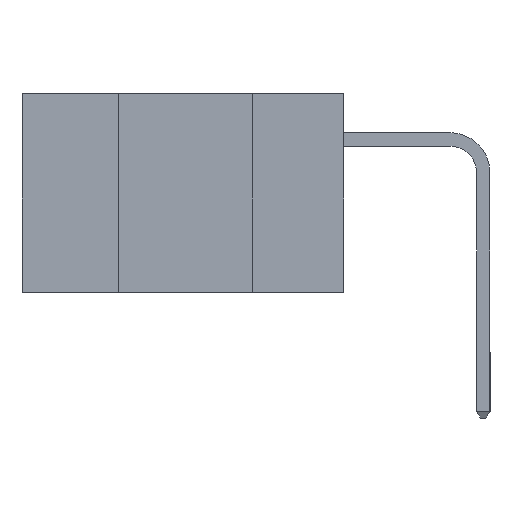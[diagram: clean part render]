
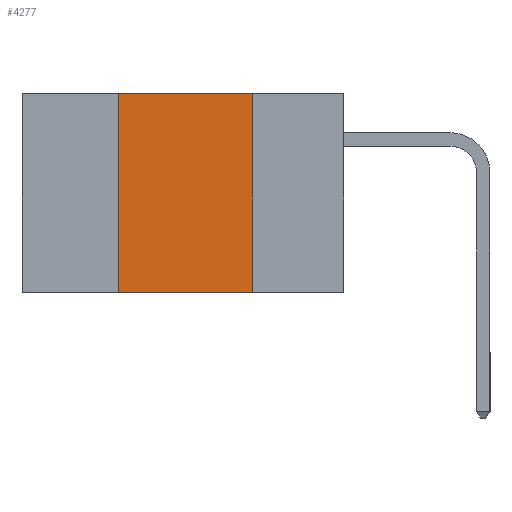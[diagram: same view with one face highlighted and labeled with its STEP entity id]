
A CAD part, left-side view. The second image highlights one B-rep face of the part: STEP entity #4277.
In plain terms, the highlighted planar face has unit normal (-1, 0, 0).
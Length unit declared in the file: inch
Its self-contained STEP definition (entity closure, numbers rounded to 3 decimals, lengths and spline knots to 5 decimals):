
#91 = LINE ( 'NONE', #2600, #12631 ) ;
#205 = EDGE_CURVE ( 'NONE', #9719, #13048, #2115, .T. ) ;
#1050 = DIRECTION ( 'NONE',  ( 0., 0., -1. ) ) ;
#1106 = CARTESIAN_POINT ( 'NONE',  ( 0., 0.17, 0. ) ) ;
#2115 = LINE ( 'NONE', #5083, #13080 ) ;
#2322 = CARTESIAN_POINT ( 'NONE',  ( 0., 0.42, 0. ) ) ;
#2352 = CARTESIAN_POINT ( 'NONE',  ( 0., 0.6, 0. ) ) ;
#2404 = DIRECTION ( 'NONE',  ( 1., 0., 0. ) ) ;
#2505 = ORIENTED_EDGE ( 'NONE', *, *, #5568, .F. ) ;
#2600 = CARTESIAN_POINT ( 'NONE',  ( 0., 0.6, 0. ) ) ;
#3003 = EDGE_CURVE ( 'NONE', #3076, #13048, #10635, .T. ) ;
#3076 = VERTEX_POINT ( 'NONE', #4480 ) ;
#3964 = CARTESIAN_POINT ( 'NONE',  ( 0., 0.42, -0.37 ) ) ;
#4085 = FACE_OUTER_BOUND ( 'NONE', #6163, .T. ) ;
#4277 = ADVANCED_FACE ( 'NONE', ( #4085 ), #10495, .F. ) ;
#4480 = CARTESIAN_POINT ( 'NONE',  ( 0., 0.17, 0. ) ) ;
#4756 = DIRECTION ( 'NONE',  ( 0., -1., 0. ) ) ;
#5083 = CARTESIAN_POINT ( 'NONE',  ( 0., 0.6, -0.37 ) ) ;
#5568 = EDGE_CURVE ( 'NONE', #8597, #3076, #91, .T. ) ;
#5594 = ORIENTED_EDGE ( 'NONE', *, *, #3003, .F. ) ;
#5931 = VECTOR ( 'NONE', #10267, 39.37008 ) ;
#6163 = EDGE_LOOP ( 'NONE', ( #5594, #2505, #7338, #10912 ) ) ;
#7194 = LINE ( 'NONE', #2322, #5931 ) ;
#7338 = ORIENTED_EDGE ( 'NONE', *, *, #8689, .F. ) ;
#7370 = DIRECTION ( 'NONE',  ( 0., -1., 0. ) ) ;
#7980 = CARTESIAN_POINT ( 'NONE',  ( 0., 0.17, -0.37 ) ) ;
#8597 = VERTEX_POINT ( 'NONE', #10981 ) ;
#8648 = VECTOR ( 'NONE', #1050, 39.37008 ) ;
#8689 = EDGE_CURVE ( 'NONE', #9719, #8597, #7194, .T. ) ;
#9719 = VERTEX_POINT ( 'NONE', #3964 ) ;
#10267 = DIRECTION ( 'NONE',  ( 0., 0., 1. ) ) ;
#10495 = PLANE ( 'NONE',  #11836 ) ;
#10635 = LINE ( 'NONE', #1106, #8648 ) ;
#10912 = ORIENTED_EDGE ( 'NONE', *, *, #205, .T. ) ;
#10981 = CARTESIAN_POINT ( 'NONE',  ( 0., 0.42, 0. ) ) ;
#11836 = AXIS2_PLACEMENT_3D ( 'NONE', #2352, #2404, #13790 ) ;
#12631 = VECTOR ( 'NONE', #7370, 39.37008 ) ;
#13048 = VERTEX_POINT ( 'NONE', #7980 ) ;
#13080 = VECTOR ( 'NONE', #4756, 39.37008 ) ;
#13790 = DIRECTION ( 'NONE',  ( 0., 0., -1. ) ) ;
